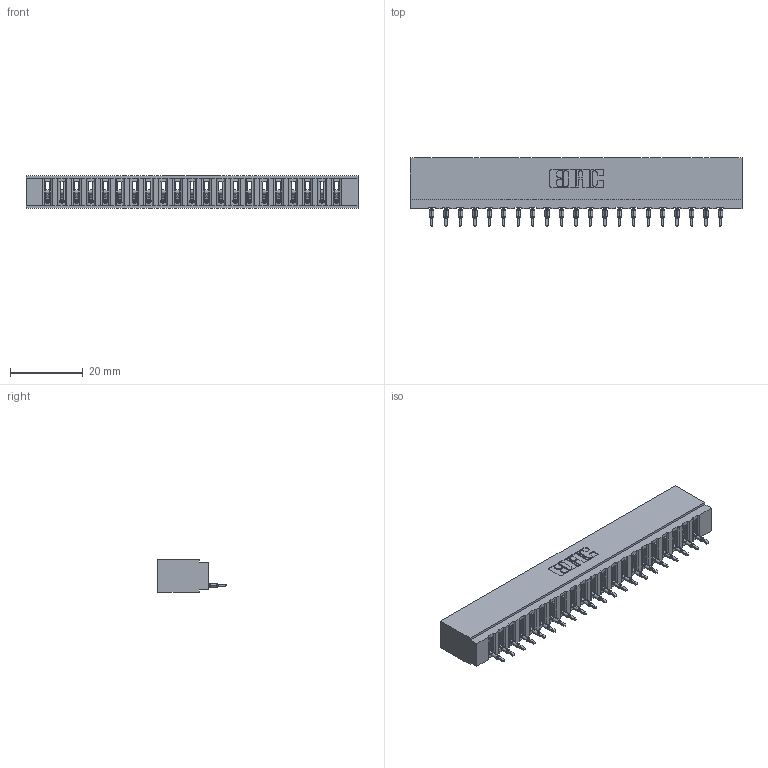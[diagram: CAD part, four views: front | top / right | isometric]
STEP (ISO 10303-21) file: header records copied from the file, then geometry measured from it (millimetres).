
FILE_DESCRIPTION (( 'STEP AP203' ), '1' );
FILE_NAME ('717-021-560-106.STEP', '2020-03-13T19:16:49', ( '' ), ( '' ), 'SwSTEP 2.0', 'SolidWorks 2016', '' );
FILE_SCHEMA (( 'CONFIG_CONTROL_DESIGN' ));
Length unit declared in the file: inch
Products named in the file (3): 745-292-001_560; 717 Part_Insulator Option - 06; 717-021-560-106
Assembly tree (22 placements, depth 2):
  717-021-560-106
    717 Part_Insulator Option - 06
    745-292-001_560  x21
Bounding box: 91.08 x 18.78 x 8.89 mm (x, y, z)
Volume: 7851.1 mm3; surface area: 11140.5 mm2
Topology: 22 solids, 22 shells, 2656 faces, 7391 edges, 4702 vertices
Faces by surface type: plane 1587, cylinder 523, bspline 420, torus 126
Entity records: 38502 total; most frequent: CARTESIAN_POINT 7288, ORIENTED_EDGE 6702, DIRECTION 5833, EDGE_CURVE 3351, LINE 3035, VECTOR 3035, VERTEX_POINT 2142, AXIS2_PLACEMENT_3D 1399
